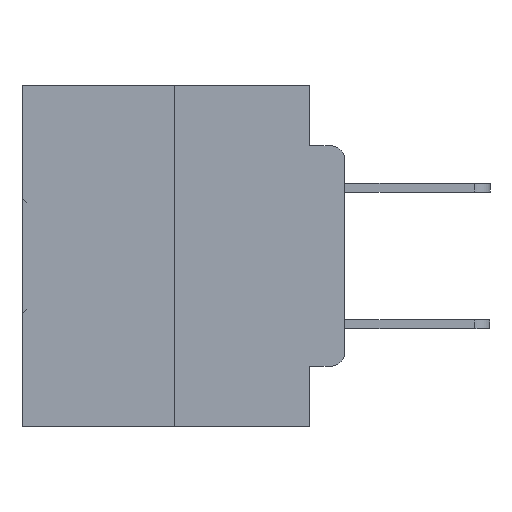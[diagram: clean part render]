
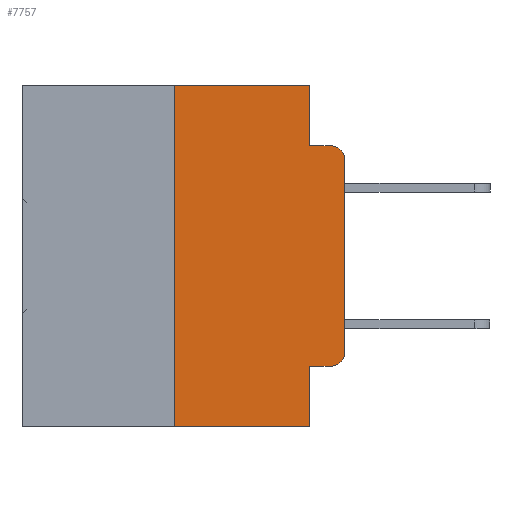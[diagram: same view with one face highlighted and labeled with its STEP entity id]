
A CAD part, left-side view. The second image highlights one B-rep face of the part: STEP entity #7757.
In plain terms, the highlighted planar face has unit normal (-1, 0, 0).
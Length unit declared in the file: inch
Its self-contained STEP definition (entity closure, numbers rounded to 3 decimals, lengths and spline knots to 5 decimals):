
#652 = CARTESIAN_POINT ( 'NONE',  ( 0., 0.25, 0. ) ) ;
#1177 = CARTESIAN_POINT ( 'NONE',  ( 0., 0.473, -0.5 ) ) ;
#1816 = VECTOR ( 'NONE', #14383, 39.37008 ) ;
#1974 = DIRECTION ( 'NONE',  ( 0., 0., -1. ) ) ;
#2345 = DIRECTION ( 'NONE',  ( 0., 0., -1. ) ) ;
#3211 = EDGE_CURVE ( 'NONE', #7810, #6286, #3380, .T. ) ;
#3321 = EDGE_CURVE ( 'NONE', #12425, #7461, #26886, .T. ) ;
#3380 = LINE ( 'NONE', #27376, #9476 ) ;
#3937 = DIRECTION ( 'NONE',  ( -1., 0., 0. ) ) ;
#4055 = ORIENTED_EDGE ( 'NONE', *, *, #26892, .F. ) ;
#4123 = VECTOR ( 'NONE', #14119, 39.37008 ) ;
#4456 = ORIENTED_EDGE ( 'NONE', *, *, #3321, .F. ) ;
#4866 = VERTEX_POINT ( 'NONE', #23214 ) ;
#5068 = ORIENTED_EDGE ( 'NONE', *, *, #19085, .T. ) ;
#5202 = LINE ( 'NONE', #10263, #11367 ) ;
#5786 = DIRECTION ( 'NONE',  ( 0., 0., 1. ) ) ;
#6028 = DIRECTION ( 'NONE',  ( 0., -1., 0. ) ) ;
#6030 = CARTESIAN_POINT ( 'NONE',  ( 0., 0.051, -0.0885 ) ) ;
#6286 = VERTEX_POINT ( 'NONE', #14301 ) ;
#7096 = ORIENTED_EDGE ( 'NONE', *, *, #18734, .T. ) ;
#7442 = VERTEX_POINT ( 'NONE', #26863 ) ;
#7461 = VERTEX_POINT ( 'NONE', #29453 ) ;
#7757 = ADVANCED_FACE ( 'NONE', ( #9934 ), #33314, .F. ) ;
#7810 = VERTEX_POINT ( 'NONE', #12942 ) ;
#8332 = EDGE_CURVE ( 'NONE', #6286, #7442, #20430, .T. ) ;
#8868 = DIRECTION ( 'NONE',  ( 0., -1., 0. ) ) ;
#9476 = VECTOR ( 'NONE', #30268, 39.37008 ) ;
#9552 = LINE ( 'NONE', #22134, #1816 ) ;
#9743 = VECTOR ( 'NONE', #19359, 39.37008 ) ;
#9934 = FACE_OUTER_BOUND ( 'NONE', #22080, .T. ) ;
#10263 = CARTESIAN_POINT ( 'NONE',  ( 0., 0., 0. ) ) ;
#10499 = AXIS2_PLACEMENT_3D ( 'NONE', #32954, #17532, #1974 ) ;
#10587 = ORIENTED_EDGE ( 'NONE', *, *, #13083, .F. ) ;
#11067 = LINE ( 'NONE', #32127, #4123 ) ;
#11367 = VECTOR ( 'NONE', #30940, 39.37008 ) ;
#11684 = VERTEX_POINT ( 'NONE', #652 ) ;
#12425 = VERTEX_POINT ( 'NONE', #6030 ) ;
#12942 = CARTESIAN_POINT ( 'NONE',  ( 0., 0.051, -0.4115 ) ) ;
#13083 = EDGE_CURVE ( 'NONE', #11684, #25763, #15751, .T. ) ;
#13545 = VERTEX_POINT ( 'NONE', #21071 ) ;
#14119 = DIRECTION ( 'NONE',  ( 0., 0., -1. ) ) ;
#14301 = CARTESIAN_POINT ( 'NONE',  ( 0., 0.02, -0.4115 ) ) ;
#14383 = DIRECTION ( 'NONE',  ( 0., 0., -1. ) ) ;
#15414 = ORIENTED_EDGE ( 'NONE', *, *, #3211, .T. ) ;
#15751 = LINE ( 'NONE', #21760, #29500 ) ;
#17532 = DIRECTION ( 'NONE',  ( -1., 0., 0. ) ) ;
#17574 = EDGE_CURVE ( 'NONE', #7810, #13545, #11067, .T. ) ;
#17696 = CARTESIAN_POINT ( 'NONE',  ( 0., 0.051, 0. ) ) ;
#17903 = DIRECTION ( 'NONE',  ( 1., 0., 0. ) ) ;
#18734 = EDGE_CURVE ( 'NONE', #29505, #13545, #22681, .T. ) ;
#18854 = AXIS2_PLACEMENT_3D ( 'NONE', #19506, #3937, #22066 ) ;
#19085 = EDGE_CURVE ( 'NONE', #7442, #4866, #5202, .T. ) ;
#19359 = DIRECTION ( 'NONE',  ( 0., -1., 0. ) ) ;
#19506 = CARTESIAN_POINT ( 'NONE',  ( 0., 0.02, -0.1085 ) ) ;
#19907 = LINE ( 'NONE', #28928, #32782 ) ;
#20308 = ORIENTED_EDGE ( 'NONE', *, *, #17574, .F. ) ;
#20430 = CIRCLE ( 'NONE', #10499, 0.02 ) ;
#20471 = AXIS2_PLACEMENT_3D ( 'NONE', #25437, #17903, #2345 ) ;
#20697 = ORIENTED_EDGE ( 'NONE', *, *, #29260, .T. ) ;
#21071 = CARTESIAN_POINT ( 'NONE',  ( 0., 0.051, -0.5 ) ) ;
#21760 = CARTESIAN_POINT ( 'NONE',  ( 0., 0.473, 0. ) ) ;
#22066 = DIRECTION ( 'NONE',  ( 0., 0., -1. ) ) ;
#22080 = EDGE_LOOP ( 'NONE', ( #5068, #20697, #4456, #29102, #10587, #4055, #7096, #20308, #15414, #27857 ) ) ;
#22134 = CARTESIAN_POINT ( 'NONE',  ( 0., 0.051, 0. ) ) ;
#22681 = LINE ( 'NONE', #1177, #9743 ) ;
#23214 = CARTESIAN_POINT ( 'NONE',  ( 0., 0., -0.1085 ) ) ;
#25437 = CARTESIAN_POINT ( 'NONE',  ( 0., 0.473, 0. ) ) ;
#25763 = VERTEX_POINT ( 'NONE', #17696 ) ;
#26054 = VECTOR ( 'NONE', #6028, 39.37008 ) ;
#26863 = CARTESIAN_POINT ( 'NONE',  ( 0., 0., -0.3915 ) ) ;
#26886 = LINE ( 'NONE', #29242, #26054 ) ;
#26892 = EDGE_CURVE ( 'NONE', #29505, #11684, #19907, .T. ) ;
#27376 = CARTESIAN_POINT ( 'NONE',  ( 0., 0.051, -0.4115 ) ) ;
#27857 = ORIENTED_EDGE ( 'NONE', *, *, #8332, .T. ) ;
#28177 = CARTESIAN_POINT ( 'NONE',  ( 0., 0.25, -0.5 ) ) ;
#28928 = CARTESIAN_POINT ( 'NONE',  ( 0., 0.25, 0. ) ) ;
#29102 = ORIENTED_EDGE ( 'NONE', *, *, #31674, .F. ) ;
#29157 = CIRCLE ( 'NONE', #18854, 0.02 ) ;
#29242 = CARTESIAN_POINT ( 'NONE',  ( 0., 0.051, -0.0885 ) ) ;
#29260 = EDGE_CURVE ( 'NONE', #4866, #7461, #29157, .T. ) ;
#29453 = CARTESIAN_POINT ( 'NONE',  ( 0., 0.02, -0.0885 ) ) ;
#29500 = VECTOR ( 'NONE', #8868, 39.37008 ) ;
#29505 = VERTEX_POINT ( 'NONE', #28177 ) ;
#30268 = DIRECTION ( 'NONE',  ( 0., -1., 0. ) ) ;
#30940 = DIRECTION ( 'NONE',  ( 0., 0., 1. ) ) ;
#31674 = EDGE_CURVE ( 'NONE', #25763, #12425, #9552, .T. ) ;
#32127 = CARTESIAN_POINT ( 'NONE',  ( 0., 0.051, 0. ) ) ;
#32782 = VECTOR ( 'NONE', #5786, 39.37008 ) ;
#32954 = CARTESIAN_POINT ( 'NONE',  ( 0., 0.02, -0.3915 ) ) ;
#33314 = PLANE ( 'NONE',  #20471 ) ;
